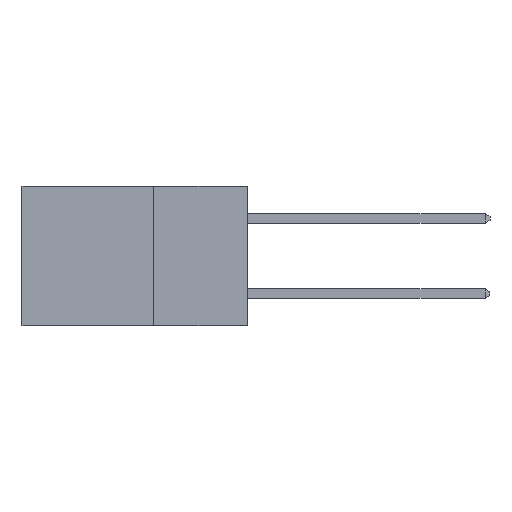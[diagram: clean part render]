
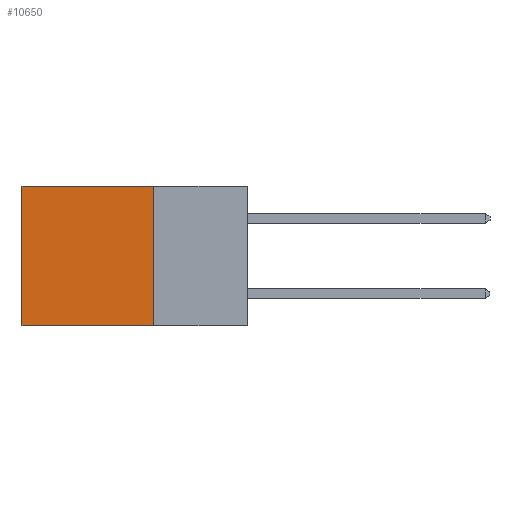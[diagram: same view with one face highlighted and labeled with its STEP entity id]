
A CAD part, left-side view. The second image highlights one B-rep face of the part: STEP entity #10650.
In plain terms, the highlighted planar face has unit normal (-1, 0, 0).
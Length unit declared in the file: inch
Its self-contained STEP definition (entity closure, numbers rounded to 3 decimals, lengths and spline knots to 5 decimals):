
#854 = VECTOR ( 'NONE', #2812, 39.37008 ) ;
#1073 = LINE ( 'NONE', #7932, #6323 ) ;
#1127 = EDGE_LOOP ( 'NONE', ( #6542, #3048, #1260, #2539 ) ) ;
#1247 = DIRECTION ( 'NONE',  ( 0., 0., -1. ) ) ;
#1260 = ORIENTED_EDGE ( 'NONE', *, *, #6941, .F. ) ;
#1923 = CARTESIAN_POINT ( 'NONE',  ( 0.298, 0.6, -0.37 ) ) ;
#2291 = VERTEX_POINT ( 'NONE', #11448 ) ;
#2539 = ORIENTED_EDGE ( 'NONE', *, *, #7724, .T. ) ;
#2636 = LINE ( 'NONE', #3183, #14174 ) ;
#2812 = DIRECTION ( 'NONE',  ( 0., 1., 0. ) ) ;
#3048 = ORIENTED_EDGE ( 'NONE', *, *, #9339, .F. ) ;
#3183 = CARTESIAN_POINT ( 'NONE',  ( 0.298, 0.25, 0. ) ) ;
#4458 = VERTEX_POINT ( 'NONE', #1923 ) ;
#5263 = DIRECTION ( 'NONE',  ( 0., 0., -1. ) ) ;
#5284 = VECTOR ( 'NONE', #1247, 39.37008 ) ;
#5420 = DIRECTION ( 'NONE',  ( 0., 0., -1. ) ) ;
#6171 = CARTESIAN_POINT ( 'NONE',  ( 0.298, 0.25, 0. ) ) ;
#6269 = VERTEX_POINT ( 'NONE', #12085 ) ;
#6323 = VECTOR ( 'NONE', #13442, 39.37008 ) ;
#6462 = LINE ( 'NONE', #10734, #854 ) ;
#6492 = EDGE_CURVE ( 'NONE', #6269, #4458, #8354, .T. ) ;
#6542 = ORIENTED_EDGE ( 'NONE', *, *, #6492, .T. ) ;
#6941 = EDGE_CURVE ( 'NONE', #10526, #2291, #2636, .T. ) ;
#6943 = AXIS2_PLACEMENT_3D ( 'NONE', #8693, #12057, #5263 ) ;
#7724 = EDGE_CURVE ( 'NONE', #10526, #6269, #1073, .T. ) ;
#7932 = CARTESIAN_POINT ( 'NONE',  ( 0.298, 0.25, 0. ) ) ;
#8354 = LINE ( 'NONE', #13516, #5284 ) ;
#8693 = CARTESIAN_POINT ( 'NONE',  ( 0.298, 0.25, 0. ) ) ;
#9339 = EDGE_CURVE ( 'NONE', #2291, #4458, #6462, .T. ) ;
#9769 = PLANE ( 'NONE',  #6943 ) ;
#10526 = VERTEX_POINT ( 'NONE', #6171 ) ;
#10650 = ADVANCED_FACE ( 'NONE', ( #12174 ), #9769, .F. ) ;
#10734 = CARTESIAN_POINT ( 'NONE',  ( 0.298, 0.25, -0.37 ) ) ;
#11448 = CARTESIAN_POINT ( 'NONE',  ( 0.298, 0.25, -0.37 ) ) ;
#12057 = DIRECTION ( 'NONE',  ( 1., 0., 0. ) ) ;
#12085 = CARTESIAN_POINT ( 'NONE',  ( 0.298, 0.6, 0. ) ) ;
#12174 = FACE_OUTER_BOUND ( 'NONE', #1127, .T. ) ;
#13442 = DIRECTION ( 'NONE',  ( 0., 1., 0. ) ) ;
#13516 = CARTESIAN_POINT ( 'NONE',  ( 0.298, 0.6, 0. ) ) ;
#14174 = VECTOR ( 'NONE', #5420, 39.37008 ) ;
